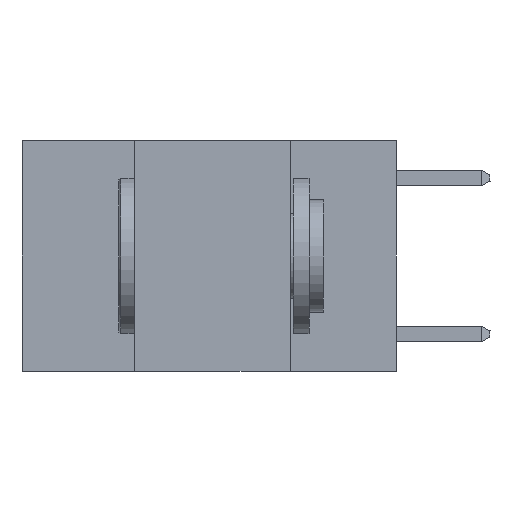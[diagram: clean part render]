
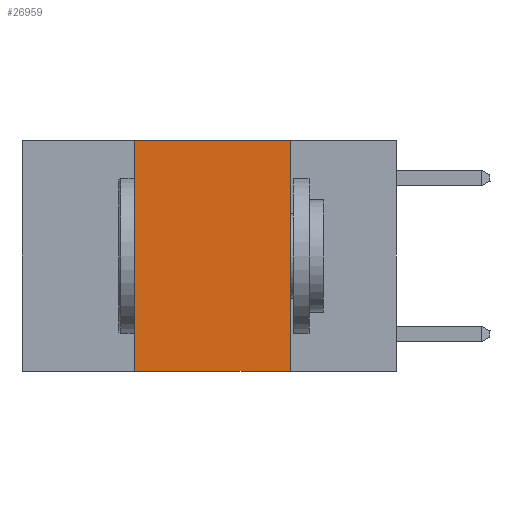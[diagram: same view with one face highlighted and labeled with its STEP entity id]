
A CAD part, left-side view. The second image highlights one B-rep face of the part: STEP entity #26959.
In plain terms, the highlighted planar face has unit normal (-1, 0, 0).
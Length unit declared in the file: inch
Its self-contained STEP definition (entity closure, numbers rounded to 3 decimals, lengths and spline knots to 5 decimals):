
#123 = ORIENTED_EDGE ( 'NONE', *, *, #30069, .F. ) ;
#652 = ORIENTED_EDGE ( 'NONE', *, *, #4833, .F. ) ;
#697 = EDGE_CURVE ( 'NONE', #20026, #21384, #7905, .T. ) ;
#4101 = DIRECTION ( 'NONE',  ( 0., -1., 0. ) ) ;
#4690 = EDGE_LOOP ( 'NONE', ( #123, #31453, #652, #17271 ) ) ;
#4833 = EDGE_CURVE ( 'NONE', #5704, #20026, #23161, .T. ) ;
#5704 = VERTEX_POINT ( 'NONE', #23589 ) ;
#7905 = LINE ( 'NONE', #22980, #12556 ) ;
#8216 = VERTEX_POINT ( 'NONE', #29364 ) ;
#8238 = DIRECTION ( 'NONE',  ( 1., 0., 0. ) ) ;
#8989 = DIRECTION ( 'NONE',  ( 0., 0., -1. ) ) ;
#8990 = LINE ( 'NONE', #16545, #11948 ) ;
#11948 = VECTOR ( 'NONE', #4101, 39.37008 ) ;
#12556 = VECTOR ( 'NONE', #18070, 39.37008 ) ;
#14476 = VECTOR ( 'NONE', #8989, 39.37008 ) ;
#15311 = CARTESIAN_POINT ( 'NONE',  ( 0., 0.42, 0. ) ) ;
#16385 = CARTESIAN_POINT ( 'NONE',  ( 0., 0.17, 0. ) ) ;
#16545 = CARTESIAN_POINT ( 'NONE',  ( 0., 0.6, -0.37 ) ) ;
#17271 = ORIENTED_EDGE ( 'NONE', *, *, #21453, .T. ) ;
#17745 = CARTESIAN_POINT ( 'NONE',  ( 0., 0.6, 0. ) ) ;
#18070 = DIRECTION ( 'NONE',  ( 0., -1., 0. ) ) ;
#18232 = DIRECTION ( 'NONE',  ( 0., 0., -1. ) ) ;
#20026 = VERTEX_POINT ( 'NONE', #24052 ) ;
#20040 = PLANE ( 'NONE',  #31617 ) ;
#20054 = DIRECTION ( 'NONE',  ( 0., 0., 1. ) ) ;
#20370 = FACE_OUTER_BOUND ( 'NONE', #4690, .T. ) ;
#21384 = VERTEX_POINT ( 'NONE', #16385 ) ;
#21453 = EDGE_CURVE ( 'NONE', #5704, #8216, #8990, .T. ) ;
#22927 = VECTOR ( 'NONE', #20054, 39.37008 ) ;
#22980 = CARTESIAN_POINT ( 'NONE',  ( 0., 0.6, 0. ) ) ;
#23161 = LINE ( 'NONE', #15311, #22927 ) ;
#23589 = CARTESIAN_POINT ( 'NONE',  ( 0., 0.42, -0.37 ) ) ;
#24052 = CARTESIAN_POINT ( 'NONE',  ( 0., 0.42, 0. ) ) ;
#24206 = CARTESIAN_POINT ( 'NONE',  ( 0., 0.17, 0. ) ) ;
#26959 = ADVANCED_FACE ( 'NONE', ( #20370 ), #20040, .F. ) ;
#28963 = LINE ( 'NONE', #24206, #14476 ) ;
#29364 = CARTESIAN_POINT ( 'NONE',  ( 0., 0.17, -0.37 ) ) ;
#30069 = EDGE_CURVE ( 'NONE', #21384, #8216, #28963, .T. ) ;
#31453 = ORIENTED_EDGE ( 'NONE', *, *, #697, .F. ) ;
#31617 = AXIS2_PLACEMENT_3D ( 'NONE', #17745, #8238, #18232 ) ;
